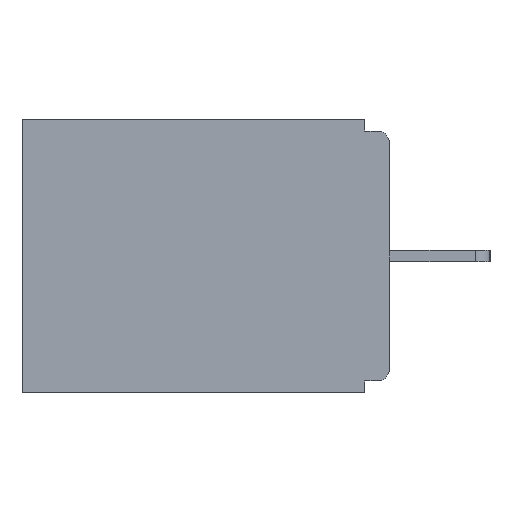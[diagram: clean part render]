
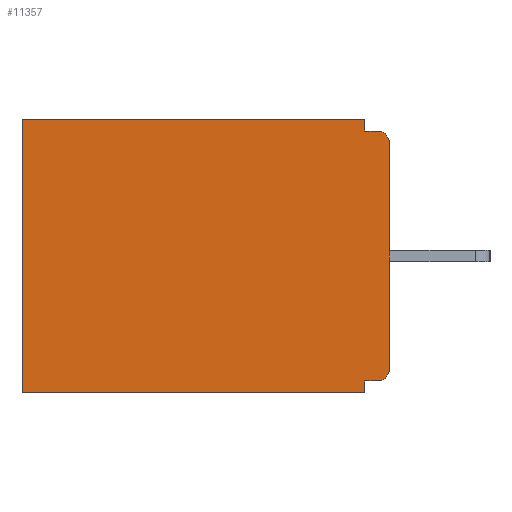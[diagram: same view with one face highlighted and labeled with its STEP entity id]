
A CAD part, left-side view. The second image highlights one B-rep face of the part: STEP entity #11357.
In plain terms, the highlighted planar face has unit normal (-1, 0, 0).
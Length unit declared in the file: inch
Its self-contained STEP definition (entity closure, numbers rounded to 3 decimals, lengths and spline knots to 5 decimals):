
#5 = VERTEX_POINT ( 'NONE', #5603 ) ;
#107 = VERTEX_POINT ( 'NONE', #12182 ) ;
#148 = VERTEX_POINT ( 'NONE', #4342 ) ;
#274 = EDGE_CURVE ( 'NONE', #7130, #5, #10932, .T. ) ;
#304 = VERTEX_POINT ( 'NONE', #5918 ) ;
#317 = DIRECTION ( 'NONE',  ( 0., 0., -1. ) ) ;
#453 = VERTEX_POINT ( 'NONE', #11653 ) ;
#813 = AXIS2_PLACEMENT_3D ( 'NONE', #9946, #9918, #6333 ) ;
#1141 = VERTEX_POINT ( 'NONE', #2393 ) ;
#1515 = DIRECTION ( 'NONE',  ( 0., 0., -1. ) ) ;
#1523 = EDGE_CURVE ( 'NONE', #304, #453, #4709, .T. ) ;
#1738 = VECTOR ( 'NONE', #7652, 39.37008 ) ;
#2050 = DIRECTION ( 'NONE',  ( 0., 1., 0. ) ) ;
#2158 = ORIENTED_EDGE ( 'NONE', *, *, #5920, .T. ) ;
#2216 = CARTESIAN_POINT ( 'NONE',  ( 0.298, 0., 0. ) ) ;
#2365 = LINE ( 'NONE', #8976, #1738 ) ;
#2393 = CARTESIAN_POINT ( 'NONE',  ( 0.298, 0., -0.313 ) ) ;
#2573 = CARTESIAN_POINT ( 'NONE',  ( 0.298, 0.031, -0.343 ) ) ;
#2614 = EDGE_CURVE ( 'NONE', #148, #1141, #9706, .T. ) ;
#2635 = EDGE_CURVE ( 'NONE', #4938, #453, #2365, .T. ) ;
#3141 = EDGE_CURVE ( 'NONE', #3378, #10341, #6225, .T. ) ;
#3378 = VERTEX_POINT ( 'NONE', #6716 ) ;
#3639 = ORIENTED_EDGE ( 'NONE', *, *, #274, .F. ) ;
#3854 = ORIENTED_EDGE ( 'NONE', *, *, #6228, .F. ) ;
#4163 = LINE ( 'NONE', #2216, #8640 ) ;
#4342 = CARTESIAN_POINT ( 'NONE',  ( 0.298, 0., -0.03 ) ) ;
#4709 = LINE ( 'NONE', #9911, #11691 ) ;
#4797 = LINE ( 'NONE', #2573, #11784 ) ;
#4938 = VERTEX_POINT ( 'NONE', #11019 ) ;
#4945 = CIRCLE ( 'NONE', #813, 0.015 ) ;
#4958 = CARTESIAN_POINT ( 'NONE',  ( 0.298, 0.031, -0.328 ) ) ;
#5124 = CARTESIAN_POINT ( 'NONE',  ( 0.298, 0.031, -0.343 ) ) ;
#5167 = DIRECTION ( 'NONE',  ( 0., 0., -1. ) ) ;
#5290 = ORIENTED_EDGE ( 'NONE', *, *, #7061, .F. ) ;
#5355 = ORIENTED_EDGE ( 'NONE', *, *, #1523, .T. ) ;
#5531 = ORIENTED_EDGE ( 'NONE', *, *, #11399, .T. ) ;
#5603 = CARTESIAN_POINT ( 'NONE',  ( 0.298, 0.031, -0.015 ) ) ;
#5661 = AXIS2_PLACEMENT_3D ( 'NONE', #9908, #9897, #9864 ) ;
#5736 = DIRECTION ( 'NONE',  ( 0., 0., -1. ) ) ;
#5763 = DIRECTION ( 'NONE',  ( -1., 0., 0. ) ) ;
#5771 = CARTESIAN_POINT ( 'NONE',  ( 0.298, 0.015, -0.313 ) ) ;
#5918 = CARTESIAN_POINT ( 'NONE',  ( 0.298, 0.46, 0. ) ) ;
#5920 = EDGE_CURVE ( 'NONE', #148, #107, #4945, .T. ) ;
#6053 = DIRECTION ( 'NONE',  ( 0., 1., 0. ) ) ;
#6156 = ORIENTED_EDGE ( 'NONE', *, *, #7695, .T. ) ;
#6225 = LINE ( 'NONE', #11385, #10732 ) ;
#6228 = EDGE_CURVE ( 'NONE', #10341, #4938, #4797, .T. ) ;
#6333 = DIRECTION ( 'NONE',  ( 0., 0., -1. ) ) ;
#6716 = CARTESIAN_POINT ( 'NONE',  ( 0.298, 0.015, -0.328 ) ) ;
#7061 = EDGE_CURVE ( 'NONE', #5, #107, #11461, .T. ) ;
#7130 = VERTEX_POINT ( 'NONE', #7910 ) ;
#7311 = PLANE ( 'NONE',  #5661 ) ;
#7321 = DIRECTION ( 'NONE',  ( 0., 0., -1. ) ) ;
#7418 = DIRECTION ( 'NONE',  ( 0., -1., 0. ) ) ;
#7652 = DIRECTION ( 'NONE',  ( 0., 1., 0. ) ) ;
#7695 = EDGE_CURVE ( 'NONE', #7130, #304, #4163, .T. ) ;
#7910 = CARTESIAN_POINT ( 'NONE',  ( 0.298, 0.031, 0. ) ) ;
#8066 = CARTESIAN_POINT ( 'NONE',  ( 0.298, 0., -0.015 ) ) ;
#8467 = VECTOR ( 'NONE', #5167, 39.37008 ) ;
#8640 = VECTOR ( 'NONE', #2050, 39.37008 ) ;
#8976 = CARTESIAN_POINT ( 'NONE',  ( 0.298, 0., -0.343 ) ) ;
#9706 = LINE ( 'NONE', #10337, #11660 ) ;
#9864 = DIRECTION ( 'NONE',  ( 0., 0., -1. ) ) ;
#9897 = DIRECTION ( 'NONE',  ( 1., 0., 0. ) ) ;
#9908 = CARTESIAN_POINT ( 'NONE',  ( 0.298, 0., 0. ) ) ;
#9911 = CARTESIAN_POINT ( 'NONE',  ( 0.298, 0.46, 0. ) ) ;
#9918 = DIRECTION ( 'NONE',  ( -1., 0., 0. ) ) ;
#9944 = EDGE_LOOP ( 'NONE', ( #2158, #5290, #3639, #6156, #5355, #10563, #3854, #12197, #5531, #10100 ) ) ;
#9946 = CARTESIAN_POINT ( 'NONE',  ( 0.298, 0.015, -0.03 ) ) ;
#10100 = ORIENTED_EDGE ( 'NONE', *, *, #2614, .F. ) ;
#10337 = CARTESIAN_POINT ( 'NONE',  ( 0.298, 0., 0. ) ) ;
#10341 = VERTEX_POINT ( 'NONE', #4958 ) ;
#10475 = AXIS2_PLACEMENT_3D ( 'NONE', #5771, #5763, #5736 ) ;
#10563 = ORIENTED_EDGE ( 'NONE', *, *, #2635, .F. ) ;
#10626 = FACE_OUTER_BOUND ( 'NONE', #9944, .T. ) ;
#10732 = VECTOR ( 'NONE', #6053, 39.37008 ) ;
#10932 = LINE ( 'NONE', #5124, #8467 ) ;
#11019 = CARTESIAN_POINT ( 'NONE',  ( 0.298, 0.031, -0.343 ) ) ;
#11151 = VECTOR ( 'NONE', #7418, 39.37008 ) ;
#11357 = ADVANCED_FACE ( 'NONE', ( #10626 ), #7311, .F. ) ;
#11385 = CARTESIAN_POINT ( 'NONE',  ( 0.298, 0., -0.328 ) ) ;
#11399 = EDGE_CURVE ( 'NONE', #3378, #1141, #11991, .T. ) ;
#11461 = LINE ( 'NONE', #8066, #11151 ) ;
#11653 = CARTESIAN_POINT ( 'NONE',  ( 0.298, 0.46, -0.343 ) ) ;
#11660 = VECTOR ( 'NONE', #1515, 39.37008 ) ;
#11691 = VECTOR ( 'NONE', #7321, 39.37008 ) ;
#11784 = VECTOR ( 'NONE', #317, 39.37008 ) ;
#11991 = CIRCLE ( 'NONE', #10475, 0.015 ) ;
#12182 = CARTESIAN_POINT ( 'NONE',  ( 0.298, 0.015, -0.015 ) ) ;
#12197 = ORIENTED_EDGE ( 'NONE', *, *, #3141, .F. ) ;
